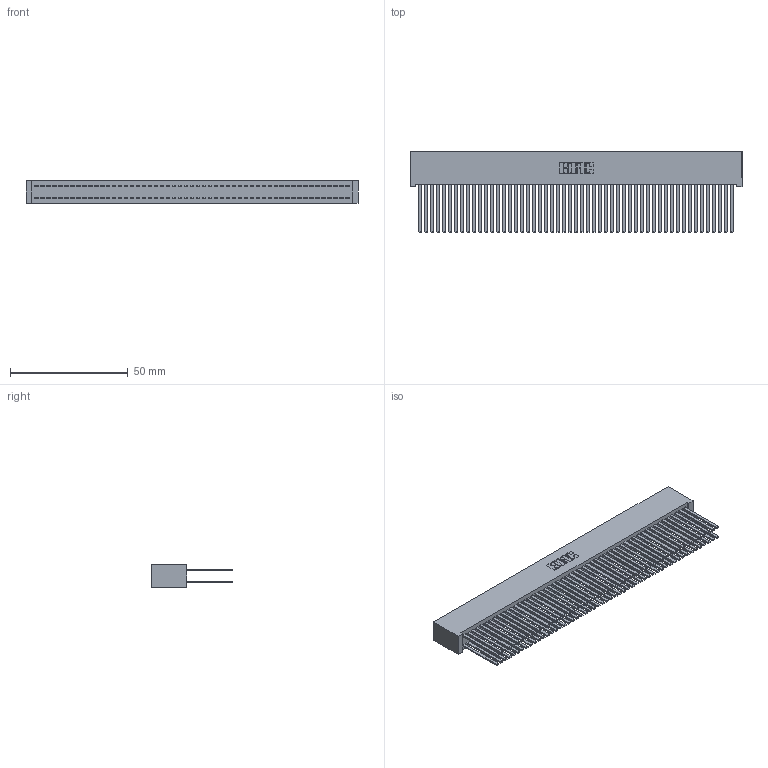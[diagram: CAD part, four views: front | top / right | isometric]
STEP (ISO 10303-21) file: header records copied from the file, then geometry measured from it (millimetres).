
FILE_DESCRIPTION (( 'STEP AP203' ), '1' );
FILE_NAME ('392-106-544-201.STEP', '2019-10-09T22:38:35', ( '' ), ( '' ), 'SwSTEP 2.0', 'SolidWorks 2016', '' );
FILE_SCHEMA (( 'CONFIG_CONTROL_DESIGN' ));
Length unit declared in the file: inch
Products named in the file (3): 342 Part_Lugless; 345-292-001_345-293-144; 392-106-544-201
Assembly tree (107 placements, depth 2):
  392-106-544-201
    342 Part_Lugless
    345-292-001_345-293-144  x106
Bounding box: 140.87 x 34.3 x 9.4 mm (x, y, z)
Volume: 14634.5 mm3; surface area: 28653.6 mm2
Topology: 107 solids, 107 shells, 4978 faces, 14797 edges, 9722 vertices
Faces by surface type: plane 3454, cylinder 1524
Entity records: 32081 total; most frequent: CARTESIAN_POINT 5298, ORIENTED_EDGE 5234, DIRECTION 4497, EDGE_CURVE 2617, VECTOR 2501, LINE 2501, VERTEX_POINT 1742, AXIS2_PLACEMENT_3D 998
